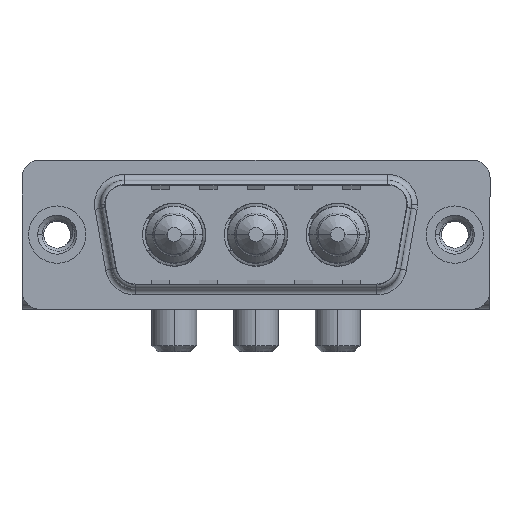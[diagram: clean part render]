
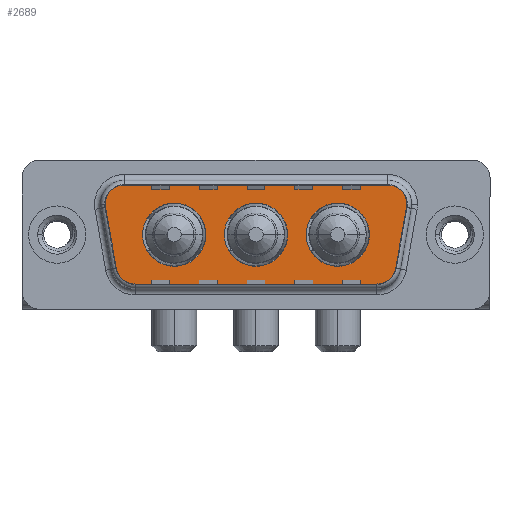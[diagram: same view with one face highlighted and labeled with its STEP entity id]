
A CAD part, top view. The second image highlights one B-rep face of the part: STEP entity #2689.
In plain terms, the highlighted planar face has unit normal (0, 0, 1).
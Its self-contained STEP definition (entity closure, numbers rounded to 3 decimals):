
#213 = ORIENTED_EDGE ( 'NONE', *, *, #8633, .F. ) ;
#293 = FACE_BOUND ( 'NONE', #4152, .T. ) ;
#303 = DIRECTION ( 'NONE',  ( 0., 0., 1. ) ) ;
#313 = DIRECTION ( 'NONE',  ( 1., 0., 0. ) ) ;
#428 = FACE_BOUND ( 'NONE', #6762, .T. ) ;
#510 = EDGE_CURVE ( 'NONE', #3257, #5433, #12240, .T. ) ;
#565 = DIRECTION ( 'NONE',  ( 0., 0., 1. ) ) ;
#675 = AXIS2_PLACEMENT_3D ( 'NONE', #12076, #565, #9806 ) ;
#705 = LINE ( 'NONE', #8094, #9800 ) ;
#854 = VERTEX_POINT ( 'NONE', #8862 ) ;
#870 = AXIS2_PLACEMENT_3D ( 'NONE', #11551, #8135, #12322 ) ;
#1072 = CARTESIAN_POINT ( 'NONE',  ( 29.859, 2.553, 0. ) ) ;
#1258 = DIRECTION ( 'NONE',  ( 0., 0., 1. ) ) ;
#1346 = CARTESIAN_POINT ( 'NONE',  ( 9.8, 0., 0. ) ) ;
#1494 = CIRCLE ( 'NONE', #13612, 2.65 ) ;
#1746 = ORIENTED_EDGE ( 'NONE', *, *, #8765, .F. ) ;
#2059 = EDGE_CURVE ( 'NONE', #2546, #11612, #3140, .T. ) ;
#2159 = AXIS2_PLACEMENT_3D ( 'NONE', #9799, #4884, #3519 ) ;
#2162 = CARTESIAN_POINT ( 'NONE',  ( 23.5, 0., 0. ) ) ;
#2244 = DIRECTION ( 'NONE',  ( 0.174, 0.985, 0. ) ) ;
#2546 = VERTEX_POINT ( 'NONE', #4355 ) ;
#2564 = CARTESIAN_POINT ( 'NONE',  ( 19.3, 0., 0. ) ) ;
#2599 = ORIENTED_EDGE ( 'NONE', *, *, #4085, .T. ) ;
#2604 = CIRCLE ( 'NONE', #9431, 2. ) ;
#2613 = VERTEX_POINT ( 'NONE', #2564 ) ;
#2689 = ADVANCED_FACE ( 'NONE', ( #293, #428, #4502, #12844 ), #3658, .T. ) ;
#2734 = ORIENTED_EDGE ( 'NONE', *, *, #9579, .T. ) ;
#3140 = LINE ( 'NONE', #1072, #8054 ) ;
#3185 = CIRCLE ( 'NONE', #12283, 2.65 ) ;
#3198 = CARTESIAN_POINT ( 'NONE',  ( 29.859, 2.553, 0. ) ) ;
#3209 = DIRECTION ( 'NONE',  ( 0., 0., 1. ) ) ;
#3257 = VERTEX_POINT ( 'NONE', #12329 ) ;
#3342 = VERTEX_POINT ( 'NONE', #11227 ) ;
#3381 = DIRECTION ( 'NONE',  ( 0., 0., 1. ) ) ;
#3434 = CARTESIAN_POINT ( 'NONE',  ( 23.5, 0., 0. ) ) ;
#3446 = EDGE_LOOP ( 'NONE', ( #5093, #12791, #6534, #2599, #9366, #4282, #7787, #2734, #3875 ) ) ;
#3519 = DIRECTION ( 'NONE',  ( -1., 0., 0. ) ) ;
#3652 = ORIENTED_EDGE ( 'NONE', *, *, #12435, .F. ) ;
#3658 = PLANE ( 'NONE',  #675 ) ;
#3691 = VERTEX_POINT ( 'NONE', #9637 ) ;
#3823 = DIRECTION ( 'NONE',  ( 0., 0., 1. ) ) ;
#3875 = ORIENTED_EDGE ( 'NONE', *, *, #510, .T. ) ;
#3957 = DIRECTION ( 'NONE',  ( 1., 0., 0. ) ) ;
#4085 = EDGE_CURVE ( 'NONE', #7857, #854, #9953, .T. ) ;
#4087 = DIRECTION ( 'NONE',  ( 1., 0., 0. ) ) ;
#4136 = CARTESIAN_POINT ( 'NONE',  ( 26.15, 0., 0. ) ) ;
#4152 = EDGE_LOOP ( 'NONE', ( #213, #3652 ) ) ;
#4282 = ORIENTED_EDGE ( 'NONE', *, *, #11486, .T. ) ;
#4297 = VERTEX_POINT ( 'NONE', #12032 ) ;
#4355 = CARTESIAN_POINT ( 'NONE',  ( 28.836, -3.247, 0. ) ) ;
#4502 = FACE_BOUND ( 'NONE', #6263, .T. ) ;
#4582 = CARTESIAN_POINT ( 'NONE',  ( 9.8, 0., 0. ) ) ;
#4623 = CARTESIAN_POINT ( 'NONE',  ( 20.85, 0., 0. ) ) ;
#4645 = AXIS2_PLACEMENT_3D ( 'NONE', #4582, #303, #5822 ) ;
#4850 = CARTESIAN_POINT ( 'NONE',  ( 26.866, -2.9, 0. ) ) ;
#4884 = DIRECTION ( 'NONE',  ( 0., 0., 1. ) ) ;
#4895 = AXIS2_PLACEMENT_3D ( 'NONE', #8196, #12388, #7161 ) ;
#5020 = EDGE_CURVE ( 'NONE', #3691, #10516, #705, .T. ) ;
#5035 = AXIS2_PLACEMENT_3D ( 'NONE', #7215, #3823, #4087 ) ;
#5093 = ORIENTED_EDGE ( 'NONE', *, *, #13272, .T. ) ;
#5126 = DIRECTION ( 'NONE',  ( 1., 0., 0. ) ) ;
#5186 = CARTESIAN_POINT ( 'NONE',  ( 26.866, -4.9, 0. ) ) ;
#5224 = AXIS2_PLACEMENT_3D ( 'NONE', #1346, #5565, #313 ) ;
#5250 = CIRCLE ( 'NONE', #2159, 2. ) ;
#5263 = DIRECTION ( 'NONE',  ( 1., 0., 0. ) ) ;
#5433 = VERTEX_POINT ( 'NONE', #5186 ) ;
#5467 = VECTOR ( 'NONE', #11860, 1000. ) ;
#5565 = DIRECTION ( 'NONE',  ( 0., 0., 1. ) ) ;
#5822 = DIRECTION ( 'NONE',  ( 1., 0., 0. ) ) ;
#5897 = CIRCLE ( 'NONE', #9853, 2.65 ) ;
#6022 = DIRECTION ( 'NONE',  ( 0.174, -0.985, 0. ) ) ;
#6073 = EDGE_CURVE ( 'NONE', #12138, #13379, #3185, .T. ) ;
#6114 = CIRCLE ( 'NONE', #5224, 2.65 ) ;
#6155 = CIRCLE ( 'NONE', #870, 2.65 ) ;
#6263 = EDGE_LOOP ( 'NONE', ( #1746, #10037 ) ) ;
#6534 = ORIENTED_EDGE ( 'NONE', *, *, #9545, .T. ) ;
#6762 = EDGE_LOOP ( 'NONE', ( #13357, #13081 ) ) ;
#7155 = CARTESIAN_POINT ( 'NONE',  ( 6.434, -4.9, 0. ) ) ;
#7161 = DIRECTION ( 'NONE',  ( -1., 0., 0. ) ) ;
#7215 = CARTESIAN_POINT ( 'NONE',  ( 5.411, 2.9, 0. ) ) ;
#7566 = CARTESIAN_POINT ( 'NONE',  ( 16.65, 0., 0. ) ) ;
#7601 = DIRECTION ( 'NONE',  ( -1., 0., 0. ) ) ;
#7787 = ORIENTED_EDGE ( 'NONE', *, *, #5020, .T. ) ;
#7857 = VERTEX_POINT ( 'NONE', #8081 ) ;
#7958 = CIRCLE ( 'NONE', #11449, 2. ) ;
#8054 = VECTOR ( 'NONE', #2244, 1000. ) ;
#8081 = CARTESIAN_POINT ( 'NONE',  ( 29.889, 2.9, 0. ) ) ;
#8094 = CARTESIAN_POINT ( 'NONE',  ( 3.441, 2.553, 0. ) ) ;
#8135 = DIRECTION ( 'NONE',  ( 0., 0., 1. ) ) ;
#8196 = CARTESIAN_POINT ( 'NONE',  ( 27.889, 2.9, 0. ) ) ;
#8633 = EDGE_CURVE ( 'NONE', #2613, #4297, #5897, .T. ) ;
#8765 = EDGE_CURVE ( 'NONE', #3342, #10365, #6114, .T. ) ;
#8826 = CIRCLE ( 'NONE', #4645, 2.65 ) ;
#8862 = CARTESIAN_POINT ( 'NONE',  ( 27.889, 4.9, 0. ) ) ;
#8911 = CARTESIAN_POINT ( 'NONE',  ( 5.411, 4.9, 0. ) ) ;
#9021 = DIRECTION ( 'NONE',  ( 1., 0., 0. ) ) ;
#9102 = EDGE_CURVE ( 'NONE', #13379, #12138, #1494, .T. ) ;
#9366 = ORIENTED_EDGE ( 'NONE', *, *, #9607, .T. ) ;
#9431 = AXIS2_PLACEMENT_3D ( 'NONE', #10760, #3381, #7601 ) ;
#9545 = EDGE_CURVE ( 'NONE', #11612, #7857, #5250, .T. ) ;
#9579 = EDGE_CURVE ( 'NONE', #10516, #3257, #2604, .T. ) ;
#9607 = EDGE_CURVE ( 'NONE', #854, #13524, #9658, .T. ) ;
#9637 = CARTESIAN_POINT ( 'NONE',  ( 3.441, 2.553, 0. ) ) ;
#9658 = LINE ( 'NONE', #13046, #5467 ) ;
#9784 = DIRECTION ( 'NONE',  ( 0., 0., 1. ) ) ;
#9799 = CARTESIAN_POINT ( 'NONE',  ( 27.889, 2.9, 0. ) ) ;
#9800 = VECTOR ( 'NONE', #6022, 1000. ) ;
#9806 = DIRECTION ( 'NONE',  ( 1., 0., 0. ) ) ;
#9853 = AXIS2_PLACEMENT_3D ( 'NONE', #7566, #3209, #10723 ) ;
#9883 = CARTESIAN_POINT ( 'NONE',  ( 4.464, -3.247, 0. ) ) ;
#9953 = CIRCLE ( 'NONE', #4895, 2. ) ;
#10037 = ORIENTED_EDGE ( 'NONE', *, *, #13080, .F. ) ;
#10365 = VERTEX_POINT ( 'NONE', #10710 ) ;
#10516 = VERTEX_POINT ( 'NONE', #9883 ) ;
#10710 = CARTESIAN_POINT ( 'NONE',  ( 7.15, 0., 0. ) ) ;
#10723 = DIRECTION ( 'NONE',  ( 1., 0., 0. ) ) ;
#10760 = CARTESIAN_POINT ( 'NONE',  ( 6.434, -2.9, 0. ) ) ;
#10974 = CIRCLE ( 'NONE', #5035, 2. ) ;
#11227 = CARTESIAN_POINT ( 'NONE',  ( 12.45, 0., 0. ) ) ;
#11449 = AXIS2_PLACEMENT_3D ( 'NONE', #4850, #13264, #5126 ) ;
#11486 = EDGE_CURVE ( 'NONE', #13524, #3691, #10974, .T. ) ;
#11517 = VECTOR ( 'NONE', #3957, 1000. ) ;
#11551 = CARTESIAN_POINT ( 'NONE',  ( 16.65, 0., 0. ) ) ;
#11612 = VERTEX_POINT ( 'NONE', #3198 ) ;
#11860 = DIRECTION ( 'NONE',  ( -1., 0., 0. ) ) ;
#12032 = CARTESIAN_POINT ( 'NONE',  ( 14., 0., 0. ) ) ;
#12076 = CARTESIAN_POINT ( 'NONE',  ( 26.866, -2.9, 0. ) ) ;
#12138 = VERTEX_POINT ( 'NONE', #4623 ) ;
#12240 = LINE ( 'NONE', #7155, #11517 ) ;
#12283 = AXIS2_PLACEMENT_3D ( 'NONE', #3434, #9784, #9021 ) ;
#12322 = DIRECTION ( 'NONE',  ( 1., 0., 0. ) ) ;
#12329 = CARTESIAN_POINT ( 'NONE',  ( 6.434, -4.9, 0. ) ) ;
#12388 = DIRECTION ( 'NONE',  ( 0., 0., 1. ) ) ;
#12435 = EDGE_CURVE ( 'NONE', #4297, #2613, #6155, .T. ) ;
#12791 = ORIENTED_EDGE ( 'NONE', *, *, #2059, .T. ) ;
#12844 = FACE_OUTER_BOUND ( 'NONE', #3446, .T. ) ;
#13046 = CARTESIAN_POINT ( 'NONE',  ( 5.411, 4.9, 0. ) ) ;
#13080 = EDGE_CURVE ( 'NONE', #10365, #3342, #8826, .T. ) ;
#13081 = ORIENTED_EDGE ( 'NONE', *, *, #6073, .F. ) ;
#13264 = DIRECTION ( 'NONE',  ( 0., 0., 1. ) ) ;
#13272 = EDGE_CURVE ( 'NONE', #5433, #2546, #7958, .T. ) ;
#13357 = ORIENTED_EDGE ( 'NONE', *, *, #9102, .F. ) ;
#13379 = VERTEX_POINT ( 'NONE', #4136 ) ;
#13524 = VERTEX_POINT ( 'NONE', #8911 ) ;
#13612 = AXIS2_PLACEMENT_3D ( 'NONE', #2162, #1258, #5263 ) ;
